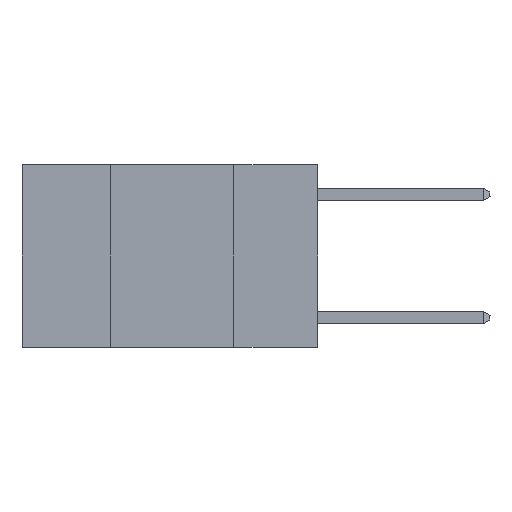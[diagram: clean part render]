
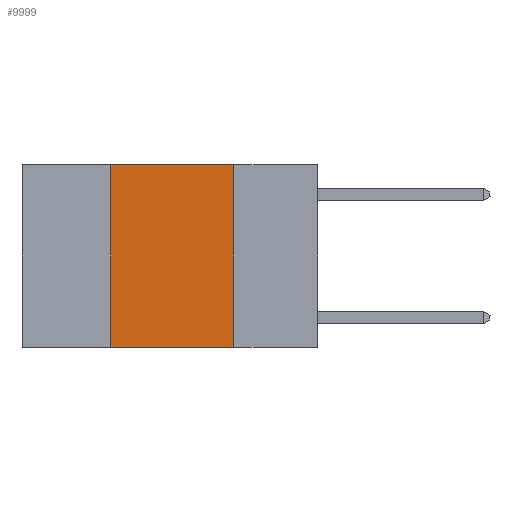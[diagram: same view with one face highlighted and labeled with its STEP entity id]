
A CAD part, left-side view. The second image highlights one B-rep face of the part: STEP entity #9999.
In plain terms, the highlighted planar face has unit normal (-1, 0, 0).
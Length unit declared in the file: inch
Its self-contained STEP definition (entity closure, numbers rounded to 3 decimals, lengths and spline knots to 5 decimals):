
#208 = DIRECTION ( 'NONE',  ( 0., -1., 0. ) ) ;
#296 = CARTESIAN_POINT ( 'NONE',  ( 0., 0.6, 0. ) ) ;
#624 = ORIENTED_EDGE ( 'NONE', *, *, #8930, .F. ) ;
#1156 = CARTESIAN_POINT ( 'NONE',  ( 0., 0.17, -0.37 ) ) ;
#1233 = EDGE_CURVE ( 'NONE', #5039, #6449, #2104, .T. ) ;
#1980 = CARTESIAN_POINT ( 'NONE',  ( 0., 0.6, 0. ) ) ;
#2104 = LINE ( 'NONE', #8528, #5679 ) ;
#2618 = VECTOR ( 'NONE', #208, 39.37008 ) ;
#3354 = ORIENTED_EDGE ( 'NONE', *, *, #6289, .T. ) ;
#3364 = CARTESIAN_POINT ( 'NONE',  ( 0., 0.17, 0. ) ) ;
#4282 = DIRECTION ( 'NONE',  ( 0., 0., -1. ) ) ;
#4648 = VERTEX_POINT ( 'NONE', #1156 ) ;
#4697 = LINE ( 'NONE', #5931, #2618 ) ;
#4798 = VECTOR ( 'NONE', #10593, 39.37008 ) ;
#4977 = CARTESIAN_POINT ( 'NONE',  ( 0., 0.17, 0. ) ) ;
#5039 = VERTEX_POINT ( 'NONE', #7692 ) ;
#5420 = EDGE_CURVE ( 'NONE', #7201, #4648, #7973, .T. ) ;
#5679 = VECTOR ( 'NONE', #11486, 39.37008 ) ;
#5931 = CARTESIAN_POINT ( 'NONE',  ( 0., 0.6, -0.37 ) ) ;
#6289 = EDGE_CURVE ( 'NONE', #5039, #4648, #4697, .T. ) ;
#6449 = VERTEX_POINT ( 'NONE', #11630 ) ;
#6524 = DIRECTION ( 'NONE',  ( 1., 0., 0. ) ) ;
#6787 = PLANE ( 'NONE',  #6818 ) ;
#6818 = AXIS2_PLACEMENT_3D ( 'NONE', #1980, #6524, #7666 ) ;
#7201 = VERTEX_POINT ( 'NONE', #3364 ) ;
#7666 = DIRECTION ( 'NONE',  ( 0., 0., -1. ) ) ;
#7692 = CARTESIAN_POINT ( 'NONE',  ( 0., 0.42, -0.37 ) ) ;
#7973 = LINE ( 'NONE', #4977, #8751 ) ;
#8528 = CARTESIAN_POINT ( 'NONE',  ( 0., 0.42, 0. ) ) ;
#8751 = VECTOR ( 'NONE', #4282, 39.37008 ) ;
#8930 = EDGE_CURVE ( 'NONE', #6449, #7201, #11474, .T. ) ;
#9616 = ORIENTED_EDGE ( 'NONE', *, *, #1233, .F. ) ;
#9999 = ADVANCED_FACE ( 'NONE', ( #11421 ), #6787, .F. ) ;
#10593 = DIRECTION ( 'NONE',  ( 0., -1., 0. ) ) ;
#11034 = EDGE_LOOP ( 'NONE', ( #11300, #624, #9616, #3354 ) ) ;
#11300 = ORIENTED_EDGE ( 'NONE', *, *, #5420, .F. ) ;
#11421 = FACE_OUTER_BOUND ( 'NONE', #11034, .T. ) ;
#11474 = LINE ( 'NONE', #296, #4798 ) ;
#11486 = DIRECTION ( 'NONE',  ( 0., 0., 1. ) ) ;
#11630 = CARTESIAN_POINT ( 'NONE',  ( 0., 0.42, 0. ) ) ;
